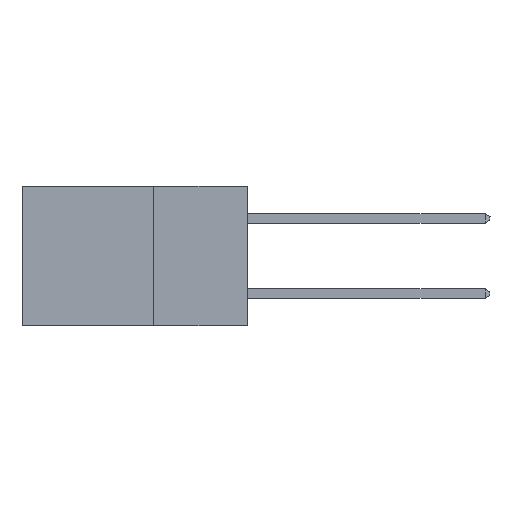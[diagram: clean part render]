
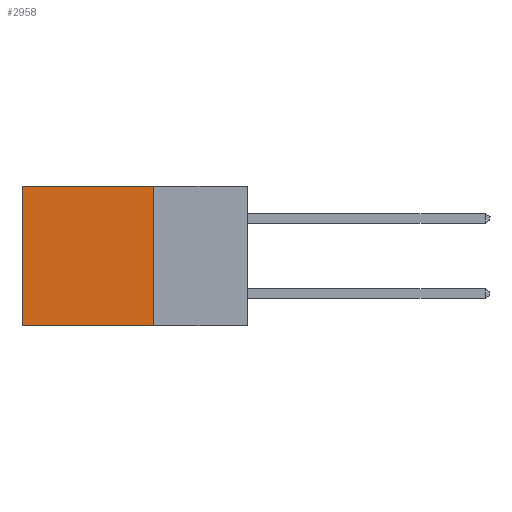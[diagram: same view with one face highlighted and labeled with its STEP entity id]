
A CAD part, left-side view. The second image highlights one B-rep face of the part: STEP entity #2958.
In plain terms, the highlighted planar face has unit normal (-1, 0, 0).
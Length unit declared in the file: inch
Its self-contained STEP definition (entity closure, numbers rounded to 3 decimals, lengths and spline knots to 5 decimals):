
#1137 = PLANE ( 'NONE',  #4511 ) ;
#2350 = LINE ( 'NONE', #13560, #4126 ) ;
#2958 = ADVANCED_FACE ( 'NONE', ( #15070 ), #1137, .F. ) ;
#2998 = VECTOR ( 'NONE', #3130, 39.37008 ) ;
#3061 = ORIENTED_EDGE ( 'NONE', *, *, #4566, .T. ) ;
#3130 = DIRECTION ( 'NONE',  ( 0., 1., 0. ) ) ;
#3514 = DIRECTION ( 'NONE',  ( 0., 0., -1. ) ) ;
#3766 = DIRECTION ( 'NONE',  ( 0., 0., -1. ) ) ;
#3831 = LINE ( 'NONE', #10195, #4523 ) ;
#4126 = VECTOR ( 'NONE', #3514, 39.37008 ) ;
#4240 = ORIENTED_EDGE ( 'NONE', *, *, #15662, .F. ) ;
#4287 = LINE ( 'NONE', #9226, #2998 ) ;
#4511 = AXIS2_PLACEMENT_3D ( 'NONE', #11525, #12684, #3766 ) ;
#4523 = VECTOR ( 'NONE', #11355, 39.37008 ) ;
#4566 = EDGE_CURVE ( 'NONE', #6906, #15579, #2350, .T. ) ;
#5842 = VERTEX_POINT ( 'NONE', #15934 ) ;
#6906 = VERTEX_POINT ( 'NONE', #12647 ) ;
#7361 = VECTOR ( 'NONE', #14421, 39.37008 ) ;
#8210 = EDGE_LOOP ( 'NONE', ( #3061, #4240, #9914, #8369 ) ) ;
#8369 = ORIENTED_EDGE ( 'NONE', *, *, #10685, .T. ) ;
#8733 = CARTESIAN_POINT ( 'NONE',  ( 0.2615, 0.6, -0.37 ) ) ;
#9226 = CARTESIAN_POINT ( 'NONE',  ( 0.2615, 0.25, -0.37 ) ) ;
#9262 = VERTEX_POINT ( 'NONE', #15741 ) ;
#9612 = LINE ( 'NONE', #14578, #7361 ) ;
#9914 = ORIENTED_EDGE ( 'NONE', *, *, #12247, .F. ) ;
#10195 = CARTESIAN_POINT ( 'NONE',  ( 0.2615, 0.25, -0.37 ) ) ;
#10685 = EDGE_CURVE ( 'NONE', #5842, #6906, #9612, .T. ) ;
#11355 = DIRECTION ( 'NONE',  ( 0., 0., -1. ) ) ;
#11525 = CARTESIAN_POINT ( 'NONE',  ( 0.2615, 0.25, -0.37 ) ) ;
#12247 = EDGE_CURVE ( 'NONE', #5842, #9262, #3831, .T. ) ;
#12647 = CARTESIAN_POINT ( 'NONE',  ( 0.2615, 0.6, 0. ) ) ;
#12684 = DIRECTION ( 'NONE',  ( 1., 0., 0. ) ) ;
#13560 = CARTESIAN_POINT ( 'NONE',  ( 0.2615, 0.6, -0.37 ) ) ;
#14421 = DIRECTION ( 'NONE',  ( 0., 1., 0. ) ) ;
#14578 = CARTESIAN_POINT ( 'NONE',  ( 0.2615, 0.25, 0. ) ) ;
#15070 = FACE_OUTER_BOUND ( 'NONE', #8210, .T. ) ;
#15579 = VERTEX_POINT ( 'NONE', #8733 ) ;
#15662 = EDGE_CURVE ( 'NONE', #9262, #15579, #4287, .T. ) ;
#15741 = CARTESIAN_POINT ( 'NONE',  ( 0.2615, 0.25, -0.37 ) ) ;
#15934 = CARTESIAN_POINT ( 'NONE',  ( 0.2615, 0.25, 0. ) ) ;
